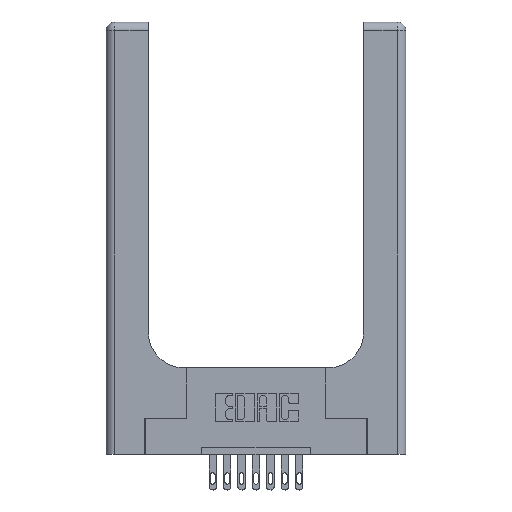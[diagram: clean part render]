
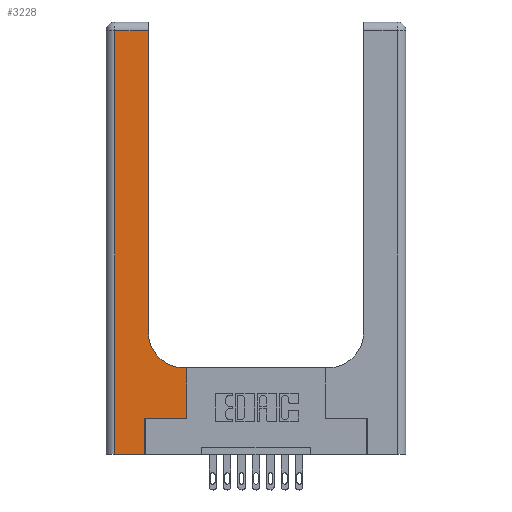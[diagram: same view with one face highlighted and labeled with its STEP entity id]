
A CAD part, top view. The second image highlights one B-rep face of the part: STEP entity #3228.
In plain terms, the highlighted planar face has unit normal (0, 0, 1).
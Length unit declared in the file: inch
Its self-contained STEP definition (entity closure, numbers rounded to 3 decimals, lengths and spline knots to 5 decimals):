
#129 = DIRECTION ( 'NONE',  ( 0., 1., 0. ) ) ;
#177 = EDGE_CURVE ( 'NONE', #12980, #4752, #9634, .T. ) ;
#268 = CARTESIAN_POINT ( 'NONE',  ( 0.2915, 0.6, 0.37 ) ) ;
#489 = DIRECTION ( 'NONE',  ( 0., 0., -1. ) ) ;
#547 = VERTEX_POINT ( 'NONE', #754 ) ;
#645 = ORIENTED_EDGE ( 'NONE', *, *, #8178, .T. ) ;
#754 = CARTESIAN_POINT ( 'NONE',  ( 0.5585, 0.25, 0.37 ) ) ;
#1013 = VECTOR ( 'NONE', #129, 39.37008 ) ;
#1293 = VERTEX_POINT ( 'NONE', #11742 ) ;
#1617 = LINE ( 'NONE', #6092, #14738 ) ;
#1864 = ORIENTED_EDGE ( 'NONE', *, *, #4147, .T. ) ;
#1867 = DIRECTION ( 'NONE',  ( 0., 1., 0. ) ) ;
#2195 = LINE ( 'NONE', #8878, #13867 ) ;
#2893 = CARTESIAN_POINT ( 'NONE',  ( 0.269, 0.25, 0.37 ) ) ;
#3007 = DIRECTION ( 'NONE',  ( 1., 0., 0. ) ) ;
#3228 = ADVANCED_FACE ( 'NONE', ( #6137 ), #14388, .F. ) ;
#3303 = CARTESIAN_POINT ( 'NONE',  ( 0.5585, 0.25, 0.37 ) ) ;
#3779 = EDGE_CURVE ( 'NONE', #4752, #547, #11778, .T. ) ;
#3914 = EDGE_CURVE ( 'NONE', #11765, #1293, #9372, .T. ) ;
#3980 = DIRECTION ( 'NONE',  ( -1., 0., 0. ) ) ;
#3996 = DIRECTION ( 'NONE',  ( 0., -1., 0. ) ) ;
#4101 = LINE ( 'NONE', #14099, #1013 ) ;
#4147 = EDGE_CURVE ( 'NONE', #7385, #12980, #1617, .T. ) ;
#4414 = VERTEX_POINT ( 'NONE', #6477 ) ;
#4606 = VECTOR ( 'NONE', #3996, 39.37008 ) ;
#4752 = VERTEX_POINT ( 'NONE', #2893 ) ;
#4953 = EDGE_CURVE ( 'NONE', #12154, #14451, #2195, .T. ) ;
#4996 = CARTESIAN_POINT ( 'NONE',  ( 0.2915, 2.94, 0.37 ) ) ;
#5155 = DIRECTION ( 'NONE',  ( 0., 1., 0. ) ) ;
#5255 = CARTESIAN_POINT ( 'NONE',  ( 0.06, 3., 0.37 ) ) ;
#5766 = ORIENTED_EDGE ( 'NONE', *, *, #13427, .T. ) ;
#5997 = EDGE_CURVE ( 'NONE', #547, #11765, #9046, .T. ) ;
#6092 = CARTESIAN_POINT ( 'NONE',  ( 0., 0., 0.37 ) ) ;
#6137 = FACE_OUTER_BOUND ( 'NONE', #8253, .T. ) ;
#6218 = DIRECTION ( 'NONE',  ( 1., 0., 0. ) ) ;
#6477 = CARTESIAN_POINT ( 'NONE',  ( 0.2915, 0.85, 0.37 ) ) ;
#6654 = DIRECTION ( 'NONE',  ( -1., 0., 0. ) ) ;
#6819 = CARTESIAN_POINT ( 'NONE',  ( 0.269, 0., 0.37 ) ) ;
#7385 = VERTEX_POINT ( 'NONE', #9835 ) ;
#7668 = LINE ( 'NONE', #5255, #4606 ) ;
#7812 = ORIENTED_EDGE ( 'NONE', *, *, #177, .T. ) ;
#8178 = EDGE_CURVE ( 'NONE', #4414, #12154, #4101, .T. ) ;
#8253 = EDGE_LOOP ( 'NONE', ( #645, #15047, #5766, #1864, #7812, #11643, #10435, #9702, #8468 ) ) ;
#8468 = ORIENTED_EDGE ( 'NONE', *, *, #9529, .T. ) ;
#8878 = CARTESIAN_POINT ( 'NONE',  ( 0., 2.94, 0.37 ) ) ;
#8980 = CARTESIAN_POINT ( 'NONE',  ( 0.269, 0.25, 0.37 ) ) ;
#9046 = LINE ( 'NONE', #3303, #9235 ) ;
#9235 = VECTOR ( 'NONE', #1867, 39.37008 ) ;
#9372 = LINE ( 'NONE', #268, #10473 ) ;
#9529 = EDGE_CURVE ( 'NONE', #1293, #4414, #11165, .T. ) ;
#9634 = LINE ( 'NONE', #9735, #14068 ) ;
#9702 = ORIENTED_EDGE ( 'NONE', *, *, #3914, .T. ) ;
#9735 = CARTESIAN_POINT ( 'NONE',  ( 0.269, 0., 0.37 ) ) ;
#9835 = CARTESIAN_POINT ( 'NONE',  ( 0.06, 0., 0.37 ) ) ;
#9991 = CARTESIAN_POINT ( 'NONE',  ( 0.5585, 0.6, 0.37 ) ) ;
#10211 = DIRECTION ( 'NONE',  ( 1., 0., 0. ) ) ;
#10435 = ORIENTED_EDGE ( 'NONE', *, *, #5997, .T. ) ;
#10473 = VECTOR ( 'NONE', #11985, 39.37008 ) ;
#10910 = CARTESIAN_POINT ( 'NONE',  ( 0., 3., 0.37 ) ) ;
#11109 = AXIS2_PLACEMENT_3D ( 'NONE', #10910, #14336, #3980 ) ;
#11165 = CIRCLE ( 'NONE', #11455, 0.25 ) ;
#11455 = AXIS2_PLACEMENT_3D ( 'NONE', #12106, #489, #6218 ) ;
#11643 = ORIENTED_EDGE ( 'NONE', *, *, #3779, .T. ) ;
#11742 = CARTESIAN_POINT ( 'NONE',  ( 0.5415, 0.6, 0.37 ) ) ;
#11765 = VERTEX_POINT ( 'NONE', #9991 ) ;
#11778 = LINE ( 'NONE', #8980, #12896 ) ;
#11985 = DIRECTION ( 'NONE',  ( -1., 0., 0. ) ) ;
#12106 = CARTESIAN_POINT ( 'NONE',  ( 0.5415, 0.85, 0.37 ) ) ;
#12154 = VERTEX_POINT ( 'NONE', #4996 ) ;
#12896 = VECTOR ( 'NONE', #10211, 39.37008 ) ;
#12980 = VERTEX_POINT ( 'NONE', #6819 ) ;
#13427 = EDGE_CURVE ( 'NONE', #14451, #7385, #7668, .T. ) ;
#13867 = VECTOR ( 'NONE', #6654, 39.37008 ) ;
#14068 = VECTOR ( 'NONE', #5155, 39.37008 ) ;
#14099 = CARTESIAN_POINT ( 'NONE',  ( 0.2915, 3., 0.37 ) ) ;
#14205 = CARTESIAN_POINT ( 'NONE',  ( 0.06, 2.94, 0.37 ) ) ;
#14336 = DIRECTION ( 'NONE',  ( 0., 0., -1. ) ) ;
#14388 = PLANE ( 'NONE',  #11109 ) ;
#14451 = VERTEX_POINT ( 'NONE', #14205 ) ;
#14738 = VECTOR ( 'NONE', #3007, 39.37008 ) ;
#15047 = ORIENTED_EDGE ( 'NONE', *, *, #4953, .T. ) ;
